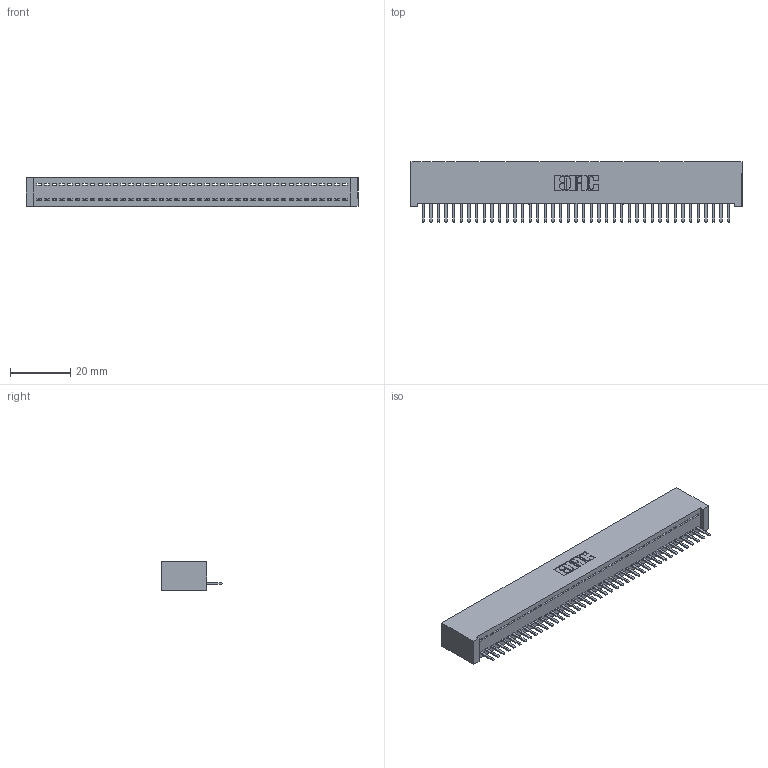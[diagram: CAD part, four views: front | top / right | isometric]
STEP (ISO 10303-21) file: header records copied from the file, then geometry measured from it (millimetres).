
FILE_DESCRIPTION (( 'STEP AP203' ), '1' );
FILE_NAME ('392-041-520-101.STEP', '2019-10-07T20:24:08', ( '' ), ( '' ), 'SwSTEP 2.0', 'SolidWorks 2016', '' );
FILE_SCHEMA (( 'CONFIG_CONTROL_DESIGN' ));
Length unit declared in the file: inch
Products named in the file (3): 345-292-001_345-293-120; 392-041-520-101; 342 Part_Lugless
Assembly tree (42 placements, depth 2):
  392-041-520-101
    342 Part_Lugless
    345-292-001_345-293-120  x41
Bounding box: 110.39 x 20.02 x 9.4 mm (x, y, z)
Volume: 9966.2 mm3; surface area: 14562.4 mm2
Topology: 42 solids, 42 shells, 2644 faces, 7819 edges, 5102 vertices
Faces by surface type: plane 1866, cylinder 778
Entity records: 24899 total; most frequent: CARTESIAN_POINT 4313, ORIENTED_EDGE 4278, DIRECTION 3621, EDGE_CURVE 2139, VECTOR 2015, LINE 2015, VERTEX_POINT 1422, AXIS2_PLACEMENT_3D 803
